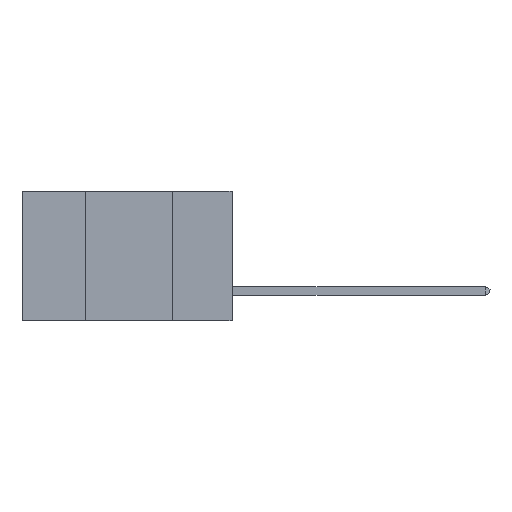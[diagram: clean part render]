
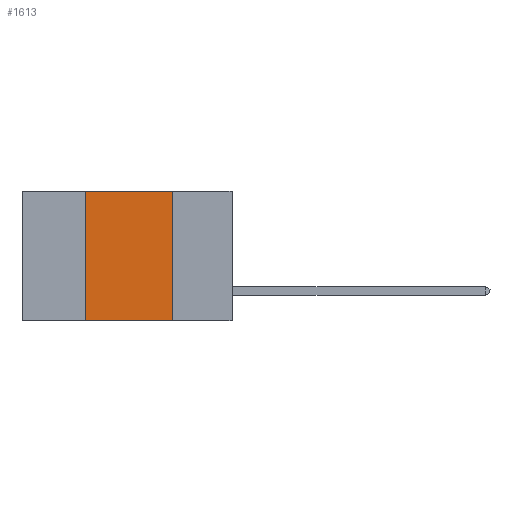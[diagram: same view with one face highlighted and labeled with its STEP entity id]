
A CAD part, left-side view. The second image highlights one B-rep face of the part: STEP entity #1613.
In plain terms, the highlighted planar face has unit normal (-1, 0, 0).
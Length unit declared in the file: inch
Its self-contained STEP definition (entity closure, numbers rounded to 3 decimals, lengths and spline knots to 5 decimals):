
#46 = ORIENTED_EDGE ( 'NONE', *, *, #5534, .F. ) ;
#701 = PLANE ( 'NONE',  #11441 ) ;
#894 = DIRECTION ( 'NONE',  ( 0., -1., 0. ) ) ;
#1461 = DIRECTION ( 'NONE',  ( 0., 0., -1. ) ) ;
#1500 = VERTEX_POINT ( 'NONE', #10598 ) ;
#1613 = ADVANCED_FACE ( 'NONE', ( #6936 ), #701, .F. ) ;
#1874 = VECTOR ( 'NONE', #2697, 39.37008 ) ;
#2415 = EDGE_LOOP ( 'NONE', ( #9989, #46, #5876, #4241 ) ) ;
#2697 = DIRECTION ( 'NONE',  ( 0., 0., 1. ) ) ;
#2738 = VECTOR ( 'NONE', #894, 39.37008 ) ;
#3471 = CARTESIAN_POINT ( 'NONE',  ( 0., 0.6, 0. ) ) ;
#4035 = EDGE_CURVE ( 'NONE', #11958, #9052, #6553, .T. ) ;
#4047 = VERTEX_POINT ( 'NONE', #7471 ) ;
#4191 = LINE ( 'NONE', #5670, #2738 ) ;
#4241 = ORIENTED_EDGE ( 'NONE', *, *, #5452, .T. ) ;
#4533 = DIRECTION ( 'NONE',  ( 0., 0., -1. ) ) ;
#4796 = CARTESIAN_POINT ( 'NONE',  ( 0., 0.6, -0.37 ) ) ;
#5452 = EDGE_CURVE ( 'NONE', #4047, #9052, #5673, .T. ) ;
#5534 = EDGE_CURVE ( 'NONE', #1500, #11958, #4191, .T. ) ;
#5670 = CARTESIAN_POINT ( 'NONE',  ( 0., 0.6, 0. ) ) ;
#5673 = LINE ( 'NONE', #4796, #10290 ) ;
#5833 = CARTESIAN_POINT ( 'NONE',  ( 0., 0.17, -0.37 ) ) ;
#5876 = ORIENTED_EDGE ( 'NONE', *, *, #6274, .F. ) ;
#6269 = VECTOR ( 'NONE', #4533, 39.37008 ) ;
#6274 = EDGE_CURVE ( 'NONE', #4047, #1500, #11683, .T. ) ;
#6553 = LINE ( 'NONE', #11013, #6269 ) ;
#6936 = FACE_OUTER_BOUND ( 'NONE', #2415, .T. ) ;
#7471 = CARTESIAN_POINT ( 'NONE',  ( 0., 0.42, -0.37 ) ) ;
#8581 = DIRECTION ( 'NONE',  ( 0., -1., 0. ) ) ;
#8664 = CARTESIAN_POINT ( 'NONE',  ( 0., 0.42, 0. ) ) ;
#8990 = DIRECTION ( 'NONE',  ( 1., 0., 0. ) ) ;
#9052 = VERTEX_POINT ( 'NONE', #5833 ) ;
#9989 = ORIENTED_EDGE ( 'NONE', *, *, #4035, .F. ) ;
#10167 = CARTESIAN_POINT ( 'NONE',  ( 0., 0.17, 0. ) ) ;
#10290 = VECTOR ( 'NONE', #8581, 39.37008 ) ;
#10598 = CARTESIAN_POINT ( 'NONE',  ( 0., 0.42, 0. ) ) ;
#11013 = CARTESIAN_POINT ( 'NONE',  ( 0., 0.17, 0. ) ) ;
#11441 = AXIS2_PLACEMENT_3D ( 'NONE', #3471, #8990, #1461 ) ;
#11683 = LINE ( 'NONE', #8664, #1874 ) ;
#11958 = VERTEX_POINT ( 'NONE', #10167 ) ;
